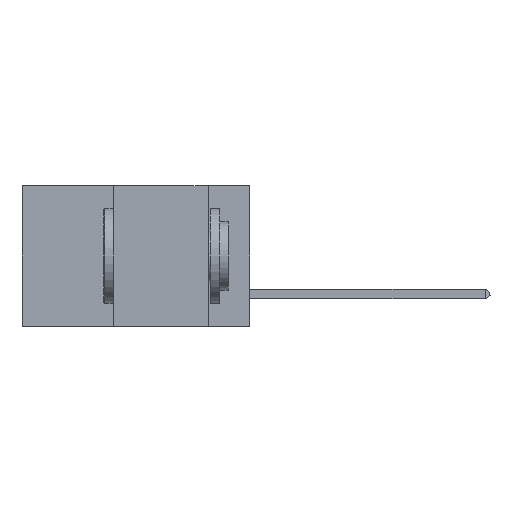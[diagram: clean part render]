
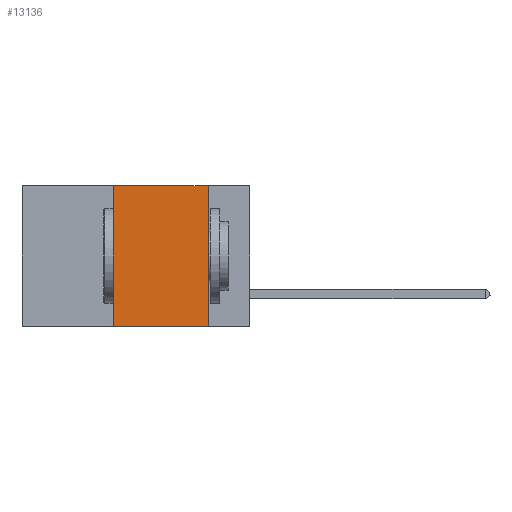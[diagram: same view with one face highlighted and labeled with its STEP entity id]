
A CAD part, left-side view. The second image highlights one B-rep face of the part: STEP entity #13136.
In plain terms, the highlighted planar face has unit normal (-1, 0, 0).
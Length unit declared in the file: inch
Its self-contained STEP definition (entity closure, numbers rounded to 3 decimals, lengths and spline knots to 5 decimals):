
#254 = FACE_OUTER_BOUND ( 'NONE', #3115, .T. ) ;
#349 = CARTESIAN_POINT ( 'NONE',  ( 0., 0.6, -0.37 ) ) ;
#535 = DIRECTION ( 'NONE',  ( 0., -1., 0. ) ) ;
#590 = EDGE_CURVE ( 'NONE', #2858, #7447, #9726, .T. ) ;
#1382 = LINE ( 'NONE', #2511, #12047 ) ;
#1522 = ORIENTED_EDGE ( 'NONE', *, *, #12482, .F. ) ;
#2310 = VECTOR ( 'NONE', #6194, 39.37008 ) ;
#2454 = ORIENTED_EDGE ( 'NONE', *, *, #6898, .F. ) ;
#2484 = PLANE ( 'NONE',  #11746 ) ;
#2511 = CARTESIAN_POINT ( 'NONE',  ( 0., 0.6, 0. ) ) ;
#2858 = VERTEX_POINT ( 'NONE', #14138 ) ;
#3071 = VECTOR ( 'NONE', #535, 39.37008 ) ;
#3115 = EDGE_LOOP ( 'NONE', ( #1522, #10999, #2454, #8169 ) ) ;
#5033 = CARTESIAN_POINT ( 'NONE',  ( 0., 0.11, 0. ) ) ;
#5385 = LINE ( 'NONE', #5033, #10093 ) ;
#5687 = CARTESIAN_POINT ( 'NONE',  ( 0., 0.6, 0. ) ) ;
#5811 = CARTESIAN_POINT ( 'NONE',  ( 0., 0.11, 0. ) ) ;
#6018 = VERTEX_POINT ( 'NONE', #5811 ) ;
#6194 = DIRECTION ( 'NONE',  ( 0., 0., 1. ) ) ;
#6334 = CARTESIAN_POINT ( 'NONE',  ( 0., 0.11, -0.37 ) ) ;
#6897 = DIRECTION ( 'NONE',  ( 0., 0., -1. ) ) ;
#6898 = EDGE_CURVE ( 'NONE', #2858, #9254, #7756, .T. ) ;
#7447 = VERTEX_POINT ( 'NONE', #6334 ) ;
#7756 = LINE ( 'NONE', #9580, #2310 ) ;
#8169 = ORIENTED_EDGE ( 'NONE', *, *, #590, .T. ) ;
#8219 = EDGE_CURVE ( 'NONE', #9254, #6018, #1382, .T. ) ;
#9254 = VERTEX_POINT ( 'NONE', #9619 ) ;
#9580 = CARTESIAN_POINT ( 'NONE',  ( 0., 0.36, 0. ) ) ;
#9619 = CARTESIAN_POINT ( 'NONE',  ( 0., 0.36, 0. ) ) ;
#9726 = LINE ( 'NONE', #349, #3071 ) ;
#10093 = VECTOR ( 'NONE', #13894, 39.37008 ) ;
#10999 = ORIENTED_EDGE ( 'NONE', *, *, #8219, .F. ) ;
#11394 = DIRECTION ( 'NONE',  ( 0., -1., 0. ) ) ;
#11746 = AXIS2_PLACEMENT_3D ( 'NONE', #5687, #13427, #6897 ) ;
#12047 = VECTOR ( 'NONE', #11394, 39.37008 ) ;
#12482 = EDGE_CURVE ( 'NONE', #6018, #7447, #5385, .T. ) ;
#13136 = ADVANCED_FACE ( 'NONE', ( #254 ), #2484, .F. ) ;
#13427 = DIRECTION ( 'NONE',  ( 1., 0., 0. ) ) ;
#13894 = DIRECTION ( 'NONE',  ( 0., 0., -1. ) ) ;
#14138 = CARTESIAN_POINT ( 'NONE',  ( 0., 0.36, -0.37 ) ) ;
